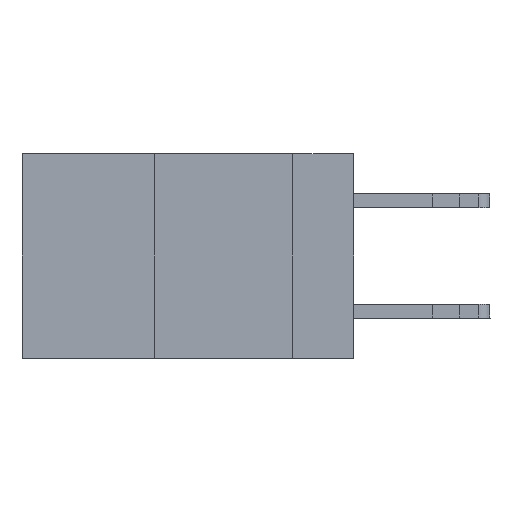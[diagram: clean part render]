
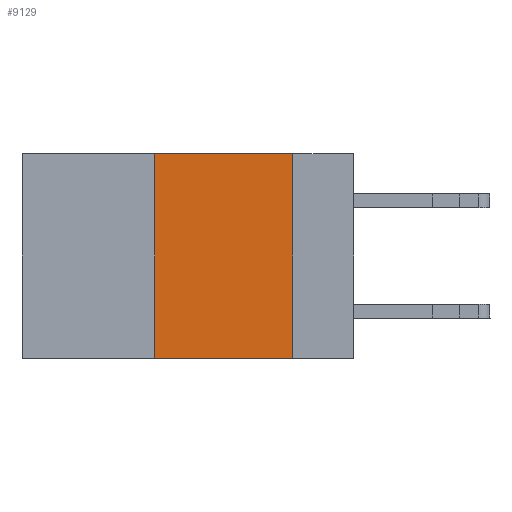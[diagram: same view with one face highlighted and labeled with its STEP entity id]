
A CAD part, left-side view. The second image highlights one B-rep face of the part: STEP entity #9129.
In plain terms, the highlighted planar face has unit normal (-1, 0, 0).
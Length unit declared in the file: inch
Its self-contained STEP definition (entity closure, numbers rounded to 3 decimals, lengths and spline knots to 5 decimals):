
#593 = PLANE ( 'NONE',  #14963 ) ;
#1288 = EDGE_CURVE ( 'NONE', #22250, #20722, #18178, .T. ) ;
#1368 = ORIENTED_EDGE ( 'NONE', *, *, #21251, .F. ) ;
#3975 = VERTEX_POINT ( 'NONE', #6859 ) ;
#4119 = DIRECTION ( 'NONE',  ( 0., 0., -1. ) ) ;
#5887 = EDGE_CURVE ( 'NONE', #22250, #3975, #7711, .T. ) ;
#6347 = DIRECTION ( 'NONE',  ( 0., -1., 0. ) ) ;
#6753 = EDGE_CURVE ( 'NONE', #12621, #20722, #12358, .T. ) ;
#6859 = CARTESIAN_POINT ( 'NONE',  ( 0., 0.36, 0. ) ) ;
#7622 = CARTESIAN_POINT ( 'NONE',  ( 0., 0.6, 0. ) ) ;
#7711 = LINE ( 'NONE', #20693, #16874 ) ;
#8179 = CARTESIAN_POINT ( 'NONE',  ( 0., 0.11, 0. ) ) ;
#8518 = VECTOR ( 'NONE', #9393, 39.37008 ) ;
#9129 = ADVANCED_FACE ( 'NONE', ( #17399 ), #593, .F. ) ;
#9393 = DIRECTION ( 'NONE',  ( 0., -1., 0. ) ) ;
#12358 = LINE ( 'NONE', #22055, #21472 ) ;
#12621 = VERTEX_POINT ( 'NONE', #8179 ) ;
#12865 = CARTESIAN_POINT ( 'NONE',  ( 0., 0.6, 0. ) ) ;
#13466 = DIRECTION ( 'NONE',  ( 0., 0., -1. ) ) ;
#13555 = VECTOR ( 'NONE', #6347, 39.37008 ) ;
#14227 = ORIENTED_EDGE ( 'NONE', *, *, #5887, .F. ) ;
#14525 = DIRECTION ( 'NONE',  ( 1., 0., 0. ) ) ;
#14963 = AXIS2_PLACEMENT_3D ( 'NONE', #12865, #14525, #4119 ) ;
#15303 = CARTESIAN_POINT ( 'NONE',  ( 0., 0.36, -0.37 ) ) ;
#15616 = EDGE_LOOP ( 'NONE', ( #18907, #1368, #14227, #16691 ) ) ;
#16691 = ORIENTED_EDGE ( 'NONE', *, *, #1288, .T. ) ;
#16874 = VECTOR ( 'NONE', #17303, 39.37008 ) ;
#17303 = DIRECTION ( 'NONE',  ( 0., 0., 1. ) ) ;
#17399 = FACE_OUTER_BOUND ( 'NONE', #15616, .T. ) ;
#17687 = LINE ( 'NONE', #7622, #8518 ) ;
#18178 = LINE ( 'NONE', #20174, #13555 ) ;
#18907 = ORIENTED_EDGE ( 'NONE', *, *, #6753, .F. ) ;
#20174 = CARTESIAN_POINT ( 'NONE',  ( 0., 0.6, -0.37 ) ) ;
#20693 = CARTESIAN_POINT ( 'NONE',  ( 0., 0.36, 0. ) ) ;
#20722 = VERTEX_POINT ( 'NONE', #22076 ) ;
#21251 = EDGE_CURVE ( 'NONE', #3975, #12621, #17687, .T. ) ;
#21472 = VECTOR ( 'NONE', #13466, 39.37008 ) ;
#22055 = CARTESIAN_POINT ( 'NONE',  ( 0., 0.11, 0. ) ) ;
#22076 = CARTESIAN_POINT ( 'NONE',  ( 0., 0.11, -0.37 ) ) ;
#22250 = VERTEX_POINT ( 'NONE', #15303 ) ;
